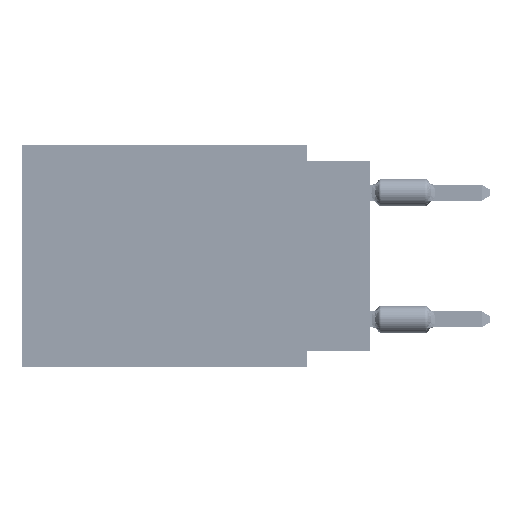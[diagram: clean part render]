
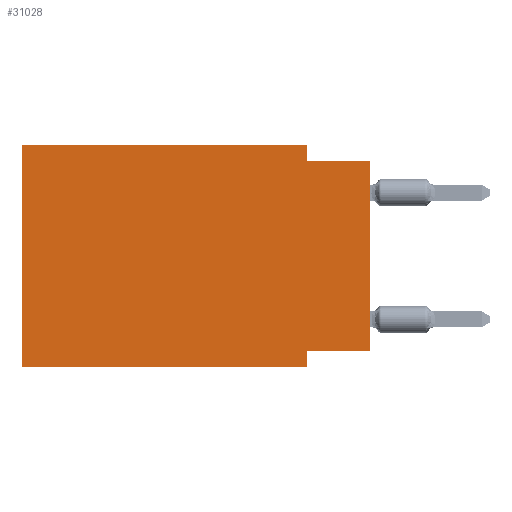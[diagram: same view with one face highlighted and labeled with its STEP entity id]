
A CAD part, left-side view. The second image highlights one B-rep face of the part: STEP entity #31028.
In plain terms, the highlighted planar face has unit normal (-1, 0, 0).
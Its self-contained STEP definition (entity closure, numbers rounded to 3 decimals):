
#537 = EDGE_CURVE ( 'NONE', #53495, #15932, #44472, .T. ) ;
#903 = DIRECTION ( 'NONE',  ( 0., 1., 0. ) ) ;
#1905 = EDGE_CURVE ( 'NONE', #14637, #15932, #67332, .T. ) ;
#2265 = EDGE_CURVE ( 'NONE', #59240, #47042, #3912, .T. ) ;
#2596 = CARTESIAN_POINT ( 'NONE',  ( 0., 2.54, 0. ) ) ;
#3298 = DIRECTION ( 'NONE',  ( 0., 0., -1. ) ) ;
#3912 = LINE ( 'NONE', #66801, #67575 ) ;
#5528 = EDGE_CURVE ( 'NONE', #5790, #47042, #7299, .T. ) ;
#5790 = VERTEX_POINT ( 'NONE', #29441 ) ;
#6650 = CARTESIAN_POINT ( 'NONE',  ( 0., 2.54, -0.635 ) ) ;
#7299 = LINE ( 'NONE', #38750, #22169 ) ;
#10837 = CARTESIAN_POINT ( 'NONE',  ( 0., 0., -0.635 ) ) ;
#11957 = ORIENTED_EDGE ( 'NONE', *, *, #47702, .F. ) ;
#12222 = LINE ( 'NONE', #43354, #19124 ) ;
#13227 = DIRECTION ( 'NONE',  ( 0., -1., 0. ) ) ;
#14637 = VERTEX_POINT ( 'NONE', #6650 ) ;
#15024 = CARTESIAN_POINT ( 'NONE',  ( 0., 0., -0.635 ) ) ;
#15225 = CARTESIAN_POINT ( 'NONE',  ( 0., 2.54, 0. ) ) ;
#15932 = VERTEX_POINT ( 'NONE', #10837 ) ;
#16201 = ORIENTED_EDGE ( 'NONE', *, *, #1905, .F. ) ;
#19124 = VECTOR ( 'NONE', #903, 1000. ) ;
#19523 = VECTOR ( 'NONE', #20489, 1000. ) ;
#20489 = DIRECTION ( 'NONE',  ( 0., -1., 0. ) ) ;
#21599 = CARTESIAN_POINT ( 'NONE',  ( 0., 2.54, -8.89 ) ) ;
#21981 = AXIS2_PLACEMENT_3D ( 'NONE', #33995, #65438, #54176 ) ;
#22169 = VECTOR ( 'NONE', #44893, 1000. ) ;
#23600 = EDGE_CURVE ( 'NONE', #30491, #37147, #33755, .T. ) ;
#24393 = CARTESIAN_POINT ( 'NONE',  ( 0., 13.97, -8.89 ) ) ;
#27637 = DIRECTION ( 'NONE',  ( 0., 0., 1. ) ) ;
#29441 = CARTESIAN_POINT ( 'NONE',  ( 0., 2.54, -8.255 ) ) ;
#29587 = LINE ( 'NONE', #49794, #61339 ) ;
#30491 = VERTEX_POINT ( 'NONE', #46487 ) ;
#30635 = EDGE_CURVE ( 'NONE', #59240, #30491, #29587, .T. ) ;
#31028 = ADVANCED_FACE ( 'NONE', ( #65770 ), #33329, .F. ) ;
#33329 = PLANE ( 'NONE',  #21981 ) ;
#33755 = LINE ( 'NONE', #54604, #44134 ) ;
#33882 = DIRECTION ( 'NONE',  ( 0., 0., 1. ) ) ;
#33995 = CARTESIAN_POINT ( 'NONE',  ( 0., 13.97, 0. ) ) ;
#34422 = ORIENTED_EDGE ( 'NONE', *, *, #66177, .F. ) ;
#34942 = EDGE_LOOP ( 'NONE', ( #51599, #16201, #11957, #46798, #59804, #43527, #53475, #34422 ) ) ;
#37147 = VERTEX_POINT ( 'NONE', #2596 ) ;
#38750 = CARTESIAN_POINT ( 'NONE',  ( 0., 2.54, -8.89 ) ) ;
#41210 = LINE ( 'NONE', #15225, #53823 ) ;
#43354 = CARTESIAN_POINT ( 'NONE',  ( 0., 0., -8.255 ) ) ;
#43527 = ORIENTED_EDGE ( 'NONE', *, *, #2265, .T. ) ;
#44134 = VECTOR ( 'NONE', #13227, 1000. ) ;
#44472 = LINE ( 'NONE', #49603, #66371 ) ;
#44893 = DIRECTION ( 'NONE',  ( 0., 0., -1. ) ) ;
#46487 = CARTESIAN_POINT ( 'NONE',  ( 0., 13.97, 0. ) ) ;
#46798 = ORIENTED_EDGE ( 'NONE', *, *, #23600, .F. ) ;
#47042 = VERTEX_POINT ( 'NONE', #21599 ) ;
#47702 = EDGE_CURVE ( 'NONE', #37147, #14637, #41210, .T. ) ;
#49603 = CARTESIAN_POINT ( 'NONE',  ( 0., 0., 0. ) ) ;
#49794 = CARTESIAN_POINT ( 'NONE',  ( 0., 13.97, 0. ) ) ;
#51599 = ORIENTED_EDGE ( 'NONE', *, *, #537, .T. ) ;
#51928 = CARTESIAN_POINT ( 'NONE',  ( 0., 0., -8.255 ) ) ;
#53475 = ORIENTED_EDGE ( 'NONE', *, *, #5528, .F. ) ;
#53495 = VERTEX_POINT ( 'NONE', #51928 ) ;
#53823 = VECTOR ( 'NONE', #3298, 1000. ) ;
#54176 = DIRECTION ( 'NONE',  ( 0., 0., -1. ) ) ;
#54604 = CARTESIAN_POINT ( 'NONE',  ( 0., 13.97, 0. ) ) ;
#59240 = VERTEX_POINT ( 'NONE', #24393 ) ;
#59804 = ORIENTED_EDGE ( 'NONE', *, *, #30635, .F. ) ;
#61339 = VECTOR ( 'NONE', #27637, 1000. ) ;
#65438 = DIRECTION ( 'NONE',  ( 1., 0., 0. ) ) ;
#65770 = FACE_OUTER_BOUND ( 'NONE', #34942, .T. ) ;
#66177 = EDGE_CURVE ( 'NONE', #53495, #5790, #12222, .T. ) ;
#66371 = VECTOR ( 'NONE', #33882, 1000. ) ;
#66801 = CARTESIAN_POINT ( 'NONE',  ( 0., 13.97, -8.89 ) ) ;
#67142 = DIRECTION ( 'NONE',  ( 0., -1., 0. ) ) ;
#67332 = LINE ( 'NONE', #15024, #19523 ) ;
#67575 = VECTOR ( 'NONE', #67142, 1000. ) ;
